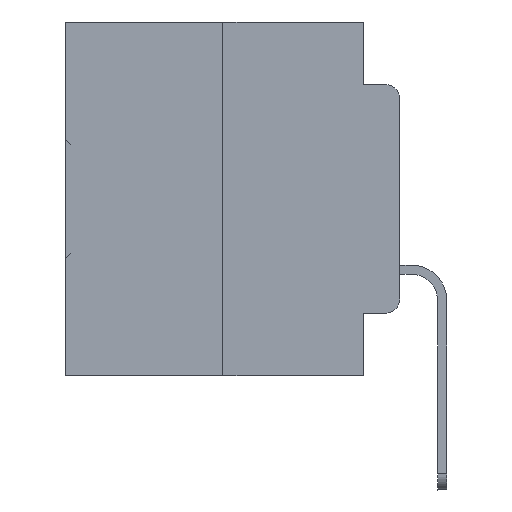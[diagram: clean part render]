
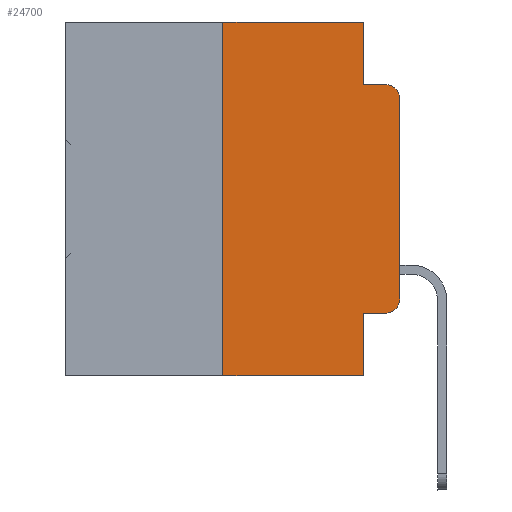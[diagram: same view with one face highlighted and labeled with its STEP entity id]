
A CAD part, left-side view. The second image highlights one B-rep face of the part: STEP entity #24700.
In plain terms, the highlighted planar face has unit normal (-1, 0, 0).
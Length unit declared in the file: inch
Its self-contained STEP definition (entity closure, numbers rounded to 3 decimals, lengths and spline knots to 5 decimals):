
#279 = DIRECTION ( 'NONE',  ( 0., -1., 0. ) ) ;
#448 = LINE ( 'NONE', #8456, #21463 ) ;
#733 = CARTESIAN_POINT ( 'NONE',  ( 0., 0.051, -0.5 ) ) ;
#1438 = LINE ( 'NONE', #14320, #5509 ) ;
#1872 = ORIENTED_EDGE ( 'NONE', *, *, #32968, .T. ) ;
#2240 = VECTOR ( 'NONE', #31304, 39.37008 ) ;
#2681 = LINE ( 'NONE', #29253, #18317 ) ;
#2791 = EDGE_CURVE ( 'NONE', #16422, #6826, #1438, .T. ) ;
#3174 = VERTEX_POINT ( 'NONE', #8546 ) ;
#3422 = CARTESIAN_POINT ( 'NONE',  ( 0., 0.02, -0.1085 ) ) ;
#4357 = DIRECTION ( 'NONE',  ( 0., 0., 1. ) ) ;
#4787 = CARTESIAN_POINT ( 'NONE',  ( 0., 0.02, -0.4115 ) ) ;
#5509 = VECTOR ( 'NONE', #17424, 39.37008 ) ;
#5593 = CARTESIAN_POINT ( 'NONE',  ( 0., 0.051, -0.4115 ) ) ;
#5617 = CARTESIAN_POINT ( 'NONE',  ( 0., 0.02, -0.3915 ) ) ;
#5684 = EDGE_CURVE ( 'NONE', #31626, #6826, #12773, .T. ) ;
#5708 = ORIENTED_EDGE ( 'NONE', *, *, #19536, .T. ) ;
#6490 = CARTESIAN_POINT ( 'NONE',  ( 0., 0.051, -0.0885 ) ) ;
#6826 = VERTEX_POINT ( 'NONE', #24434 ) ;
#7737 = ORIENTED_EDGE ( 'NONE', *, *, #12092, .T. ) ;
#8067 = ORIENTED_EDGE ( 'NONE', *, *, #2791, .F. ) ;
#8429 = VECTOR ( 'NONE', #27553, 39.37008 ) ;
#8456 = CARTESIAN_POINT ( 'NONE',  ( 0., 0.473, -0.5 ) ) ;
#8546 = CARTESIAN_POINT ( 'NONE',  ( 0., 0., -0.3915 ) ) ;
#8571 = LINE ( 'NONE', #24521, #19761 ) ;
#8640 = VERTEX_POINT ( 'NONE', #733 ) ;
#8813 = DIRECTION ( 'NONE',  ( 0., 0., -1. ) ) ;
#9181 = VECTOR ( 'NONE', #29593, 39.37008 ) ;
#9582 = LINE ( 'NONE', #27974, #33867 ) ;
#10147 = VERTEX_POINT ( 'NONE', #5593 ) ;
#11156 = DIRECTION ( 'NONE',  ( 0., 0., -1. ) ) ;
#11400 = EDGE_CURVE ( 'NONE', #27883, #16637, #2681, .T. ) ;
#11425 = VERTEX_POINT ( 'NONE', #4787 ) ;
#11782 = EDGE_CURVE ( 'NONE', #16637, #23271, #23137, .T. ) ;
#12092 = EDGE_CURVE ( 'NONE', #3174, #31626, #9582, .T. ) ;
#12354 = AXIS2_PLACEMENT_3D ( 'NONE', #12391, #15679, #25919 ) ;
#12391 = CARTESIAN_POINT ( 'NONE',  ( 0., 0.473, 0. ) ) ;
#12773 = CIRCLE ( 'NONE', #21620, 0.02 ) ;
#12782 = EDGE_CURVE ( 'NONE', #27883, #8640, #448, .T. ) ;
#12908 = CARTESIAN_POINT ( 'NONE',  ( 0., 0.473, 0. ) ) ;
#13276 = LINE ( 'NONE', #31840, #9181 ) ;
#13291 = DIRECTION ( 'NONE',  ( 0., 0., 1. ) ) ;
#13765 = CARTESIAN_POINT ( 'NONE',  ( 0., 0.25, -0.5 ) ) ;
#14320 = CARTESIAN_POINT ( 'NONE',  ( 0., 0.051, -0.0885 ) ) ;
#14986 = ORIENTED_EDGE ( 'NONE', *, *, #5684, .T. ) ;
#15153 = CARTESIAN_POINT ( 'NONE',  ( 0., 0.25, 0. ) ) ;
#15342 = PLANE ( 'NONE',  #12354 ) ;
#15679 = DIRECTION ( 'NONE',  ( 1., 0., 0. ) ) ;
#15952 = AXIS2_PLACEMENT_3D ( 'NONE', #5617, #32677, #11156 ) ;
#16339 = ORIENTED_EDGE ( 'NONE', *, *, #12782, .T. ) ;
#16422 = VERTEX_POINT ( 'NONE', #6490 ) ;
#16637 = VERTEX_POINT ( 'NONE', #15153 ) ;
#17082 = ORIENTED_EDGE ( 'NONE', *, *, #22627, .F. ) ;
#17424 = DIRECTION ( 'NONE',  ( 0., -1., 0. ) ) ;
#17555 = ORIENTED_EDGE ( 'NONE', *, *, #30568, .F. ) ;
#18317 = VECTOR ( 'NONE', #13291, 39.37008 ) ;
#18887 = CARTESIAN_POINT ( 'NONE',  ( 0., 0.051, 0. ) ) ;
#19536 = EDGE_CURVE ( 'NONE', #10147, #11425, #24427, .T. ) ;
#19761 = VECTOR ( 'NONE', #27306, 39.37008 ) ;
#20533 = FACE_OUTER_BOUND ( 'NONE', #30319, .T. ) ;
#21463 = VECTOR ( 'NONE', #279, 39.37008 ) ;
#21620 = AXIS2_PLACEMENT_3D ( 'NONE', #3422, #26865, #8813 ) ;
#22627 = EDGE_CURVE ( 'NONE', #23271, #16422, #13276, .T. ) ;
#23137 = LINE ( 'NONE', #12908, #2240 ) ;
#23271 = VERTEX_POINT ( 'NONE', #18887 ) ;
#23316 = CARTESIAN_POINT ( 'NONE',  ( 0., 0., -0.1085 ) ) ;
#24427 = LINE ( 'NONE', #32594, #8429 ) ;
#24434 = CARTESIAN_POINT ( 'NONE',  ( 0., 0.02, -0.0885 ) ) ;
#24521 = CARTESIAN_POINT ( 'NONE',  ( 0., 0.051, 0. ) ) ;
#24700 = ADVANCED_FACE ( 'NONE', ( #20533 ), #15342, .F. ) ;
#25919 = DIRECTION ( 'NONE',  ( 0., 0., -1. ) ) ;
#25950 = CIRCLE ( 'NONE', #15952, 0.02 ) ;
#26865 = DIRECTION ( 'NONE',  ( -1., 0., 0. ) ) ;
#27306 = DIRECTION ( 'NONE',  ( 0., 0., -1. ) ) ;
#27553 = DIRECTION ( 'NONE',  ( 0., -1., 0. ) ) ;
#27883 = VERTEX_POINT ( 'NONE', #13765 ) ;
#27974 = CARTESIAN_POINT ( 'NONE',  ( 0., 0., 0. ) ) ;
#29253 = CARTESIAN_POINT ( 'NONE',  ( 0., 0.25, 0. ) ) ;
#29593 = DIRECTION ( 'NONE',  ( 0., 0., -1. ) ) ;
#30319 = EDGE_LOOP ( 'NONE', ( #7737, #14986, #8067, #17082, #30856, #32860, #16339, #17555, #5708, #1872 ) ) ;
#30568 = EDGE_CURVE ( 'NONE', #10147, #8640, #8571, .T. ) ;
#30856 = ORIENTED_EDGE ( 'NONE', *, *, #11782, .F. ) ;
#31304 = DIRECTION ( 'NONE',  ( 0., -1., 0. ) ) ;
#31626 = VERTEX_POINT ( 'NONE', #23316 ) ;
#31840 = CARTESIAN_POINT ( 'NONE',  ( 0., 0.051, 0. ) ) ;
#32594 = CARTESIAN_POINT ( 'NONE',  ( 0., 0.051, -0.4115 ) ) ;
#32677 = DIRECTION ( 'NONE',  ( -1., 0., 0. ) ) ;
#32860 = ORIENTED_EDGE ( 'NONE', *, *, #11400, .F. ) ;
#32968 = EDGE_CURVE ( 'NONE', #11425, #3174, #25950, .T. ) ;
#33867 = VECTOR ( 'NONE', #4357, 39.37008 ) ;
